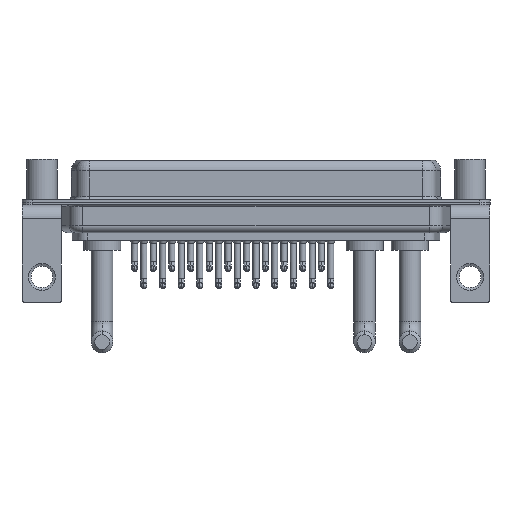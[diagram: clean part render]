
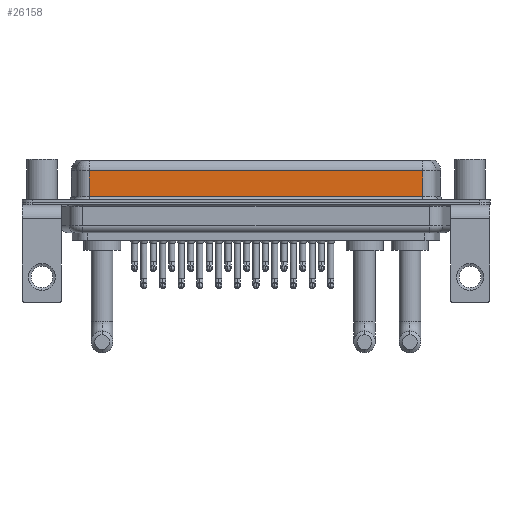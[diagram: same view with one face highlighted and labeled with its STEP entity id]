
A CAD part, front view. The second image highlights one B-rep face of the part: STEP entity #26158.
In plain terms, the highlighted planar face has unit normal (0, -1, 0).
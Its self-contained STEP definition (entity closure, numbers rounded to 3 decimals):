
#239 = FACE_OUTER_BOUND ( 'NONE', #22502, .T. ) ;
#368 = PLANE ( 'NONE',  #2747 ) ;
#603 = VECTOR ( 'NONE', #24092, 1000. ) ;
#1451 = VERTEX_POINT ( 'NONE', #9561 ) ;
#1621 = ORIENTED_EDGE ( 'NONE', *, *, #24641, .T. ) ;
#1705 = ORIENTED_EDGE ( 'NONE', *, *, #7361, .T. ) ;
#2223 = CARTESIAN_POINT ( 'NONE',  ( 56.462, -3.95, 0.9 ) ) ;
#2375 = VECTOR ( 'NONE', #11900, 1000. ) ;
#2747 = AXIS2_PLACEMENT_3D ( 'NONE', #8511, #5966, #8384 ) ;
#3613 = ORIENTED_EDGE ( 'NONE', *, *, #23535, .T. ) ;
#4722 = LINE ( 'NONE', #25112, #21840 ) ;
#5966 = DIRECTION ( 'NONE',  ( 0., 1., 0. ) ) ;
#6897 = CARTESIAN_POINT ( 'NONE',  ( 56.462, -3.95, 0.9 ) ) ;
#7361 = EDGE_CURVE ( 'NONE', #17477, #10400, #20191, .T. ) ;
#7370 = LINE ( 'NONE', #13503, #2375 ) ;
#8384 = DIRECTION ( 'NONE',  ( 0., 0., 1. ) ) ;
#8511 = CARTESIAN_POINT ( 'NONE',  ( 56.462, -3.95, 6.4 ) ) ;
#9375 = VECTOR ( 'NONE', #24047, 1000. ) ;
#9561 = CARTESIAN_POINT ( 'NONE',  ( 7.038, -3.95, 0.9 ) ) ;
#10400 = VERTEX_POINT ( 'NONE', #24026 ) ;
#10866 = DIRECTION ( 'NONE',  ( 0., 0., -1. ) ) ;
#11380 = CARTESIAN_POINT ( 'NONE',  ( 56.462, -3.95, 4.65 ) ) ;
#11689 = VERTEX_POINT ( 'NONE', #6897 ) ;
#11900 = DIRECTION ( 'NONE',  ( 0., 0., -1. ) ) ;
#13503 = CARTESIAN_POINT ( 'NONE',  ( 56.462, -3.95, 6.4 ) ) ;
#15081 = ORIENTED_EDGE ( 'NONE', *, *, #17534, .F. ) ;
#17477 = VERTEX_POINT ( 'NONE', #11380 ) ;
#17534 = EDGE_CURVE ( 'NONE', #17477, #11689, #7370, .T. ) ;
#18097 = LINE ( 'NONE', #2223, #603 ) ;
#20191 = LINE ( 'NONE', #24317, #9375 ) ;
#21840 = VECTOR ( 'NONE', #10866, 1000. ) ;
#22502 = EDGE_LOOP ( 'NONE', ( #15081, #1705, #3613, #1621 ) ) ;
#23535 = EDGE_CURVE ( 'NONE', #10400, #1451, #4722, .T. ) ;
#24026 = CARTESIAN_POINT ( 'NONE',  ( 7.038, -3.95, 4.65 ) ) ;
#24047 = DIRECTION ( 'NONE',  ( -1., 0., 0. ) ) ;
#24092 = DIRECTION ( 'NONE',  ( 1., 0., 0. ) ) ;
#24317 = CARTESIAN_POINT ( 'NONE',  ( 56.462, -3.95, 4.65 ) ) ;
#24641 = EDGE_CURVE ( 'NONE', #1451, #11689, #18097, .T. ) ;
#25112 = CARTESIAN_POINT ( 'NONE',  ( 7.038, -3.95, 6.4 ) ) ;
#26158 = ADVANCED_FACE ( 'NONE', ( #239 ), #368, .F. ) ;
